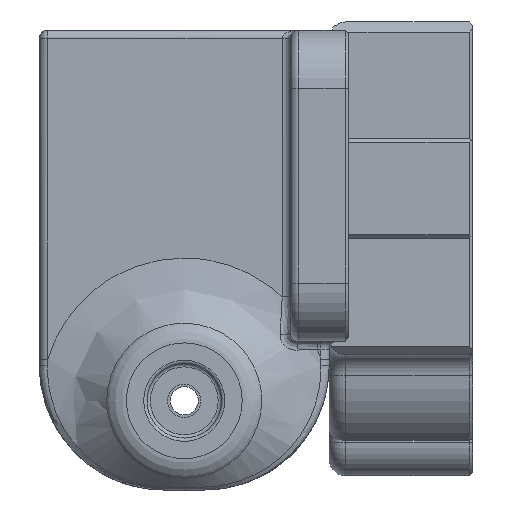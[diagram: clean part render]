
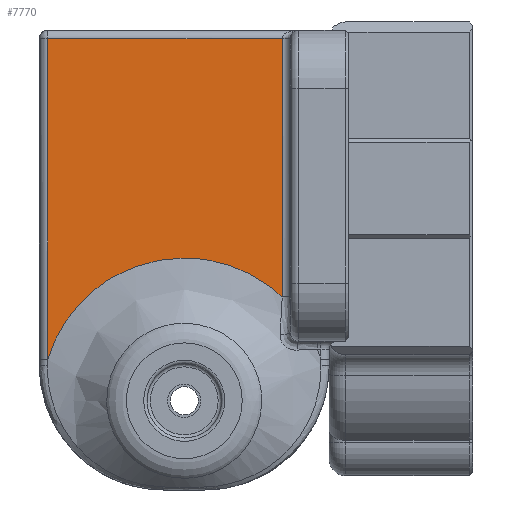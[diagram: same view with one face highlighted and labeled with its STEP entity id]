
A CAD part, front view. The second image highlights one B-rep face of the part: STEP entity #7770.
In plain terms, the highlighted planar face has unit normal (0, -1, 0).
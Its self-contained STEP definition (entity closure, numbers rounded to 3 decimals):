
#4 = EDGE_CURVE ( 'NONE', #7866, #7392, #4444, .T. ) ;
#125 = DIRECTION ( 'NONE',  ( 0., 0., 1. ) ) ;
#129 = LINE ( 'NONE', #6286, #3605 ) ;
#166 = B_SPLINE_CURVE_WITH_KNOTS ( 'NONE', 3,
 ( #6291, #770, #1392, #2013, #3269, #1982 ),
 .UNSPECIFIED., .F., .F.,
 ( 4, 1, 1, 4 ),
 ( -1.112, -0.768, -0.383, 0.001 ),
 .UNSPECIFIED. ) ;
#268 = DIRECTION ( 'NONE',  ( 0., 0., -1. ) ) ;
#488 = VERTEX_POINT ( 'NONE', #605 ) ;
#605 = CARTESIAN_POINT ( 'NONE',  ( -230.016, -0.918, 19.1 ) ) ;
#711 = DIRECTION ( 'NONE',  ( 0., 1., 0. ) ) ;
#770 = CARTESIAN_POINT ( 'NONE',  ( -204.019, -0.918, -10.226 ) ) ;
#774 = CARTESIAN_POINT ( 'NONE',  ( -222.019, -0.918, -9.62 ) ) ;
#786 = FACE_OUTER_BOUND ( 'NONE', #4139, .T. ) ;
#806 = CARTESIAN_POINT ( 'NONE',  ( -216.108, -0.918, -7.422 ) ) ;
#921 = CARTESIAN_POINT ( 'NONE',  ( -201.682, -0.918, 19.1 ) ) ;
#1008 = ORIENTED_EDGE ( 'NONE', *, *, #7106, .F. ) ;
#1229 = EDGE_CURVE ( 'NONE', #7392, #1344, #7686, .T. ) ;
#1278 = DIRECTION ( 'NONE',  ( -1., 0., 0. ) ) ;
#1291 = VERTEX_POINT ( 'NONE', #7319 ) ;
#1344 = VERTEX_POINT ( 'NONE', #6747 ) ;
#1392 = CARTESIAN_POINT ( 'NONE',  ( -206.115, -0.918, -8.942 ) ) ;
#1719 = CARTESIAN_POINT ( 'NONE',  ( -225.172, -0.918, -11.883 ) ) ;
#1823 = CARTESIAN_POINT ( 'NONE',  ( -230.014, -0.918, -19.646 ) ) ;
#1982 = CARTESIAN_POINT ( 'NONE',  ( -213.533, -0.918, -7.42 ) ) ;
#2013 = CARTESIAN_POINT ( 'NONE',  ( -209.663, -0.918, -7.708 ) ) ;
#2102 = CARTESIAN_POINT ( 'NONE',  ( -201.682, -0.918, 8.994 ) ) ;
#2452 = CARTESIAN_POINT ( 'NONE',  ( -223.933, -0.918, -10.924 ) ) ;
#2683 = CARTESIAN_POINT ( 'NONE',  ( -223.011, -0.918, -10.226 ) ) ;
#3020 = CARTESIAN_POINT ( 'NONE',  ( -224.042, -0.918, -11.007 ) ) ;
#3093 = ORIENTED_EDGE ( 'NONE', *, *, #7753, .F. ) ;
#3113 = CARTESIAN_POINT ( 'NONE',  ( -201.682, -0.918, -12.122 ) ) ;
#3269 = CARTESIAN_POINT ( 'NONE',  ( -212.247, -0.918, -7.419 ) ) ;
#3275 = LINE ( 'NONE', #2102, #5748 ) ;
#3421 = CARTESIAN_POINT ( 'NONE',  ( -213.533, -0.918, -7.42 ) ) ;
#3543 = CARTESIAN_POINT ( 'NONE',  ( -229.378, -0.918, -17.565 ) ) ;
#3586 = ORIENTED_EDGE ( 'NONE', *, *, #1229, .F. ) ;
#3605 = VECTOR ( 'NONE', #125, 1000. ) ;
#3627 = DIRECTION ( 'NONE',  ( 1., 0., 0. ) ) ;
#3890 = VERTEX_POINT ( 'NONE', #921 ) ;
#4108 = ORIENTED_EDGE ( 'NONE', *, *, #4, .F. ) ;
#4139 = EDGE_LOOP ( 'NONE', ( #4425, #5454, #3093, #3586, #4108, #1008, #6255 ) ) ;
#4283 = EDGE_CURVE ( 'NONE', #1291, #7085, #7699, .T. ) ;
#4379 = CARTESIAN_POINT ( 'NONE',  ( -203.098, -0.918, -10.924 ) ) ;
#4425 = ORIENTED_EDGE ( 'NONE', *, *, #6839, .F. ) ;
#4444 = B_SPLINE_CURVE_WITH_KNOTS ( 'NONE', 3,
 ( #7553, #806, #4451, #774, #2683, #5092 ),
 .UNSPECIFIED., .F., .F.,
 ( 4, 2, 4 ),
 ( 0.002, 0.771, 1.115 ),
 .UNSPECIFIED. ) ;
#4451 = CARTESIAN_POINT ( 'NONE',  ( -218.658, -0.918, -8.005 ) ) ;
#4852 = CARTESIAN_POINT ( 'NONE',  ( -228.349, -0.918, -15.606 ) ) ;
#4931 = CARTESIAN_POINT ( 'NONE',  ( -202.605, -0.918, -11.298 ) ) ;
#5059 = CARTESIAN_POINT ( 'NONE',  ( -203.098, -0.918, -10.924 ) ) ;
#5092 = CARTESIAN_POINT ( 'NONE',  ( -223.933, -0.918, -10.924 ) ) ;
#5295 = LINE ( 'NONE', #5438, #6354 ) ;
#5408 = CARTESIAN_POINT ( 'NONE',  ( -226.188, -0.918, -12.897 ) ) ;
#5438 = CARTESIAN_POINT ( 'NONE',  ( -213.516, -0.918, 19.1 ) ) ;
#5454 = ORIENTED_EDGE ( 'NONE', *, *, #6312, .F. ) ;
#5591 = PLANE ( 'NONE',  #5992 ) ;
#5748 = VECTOR ( 'NONE', #268, 1000. ) ;
#5848 = CARTESIAN_POINT ( 'NONE',  ( -223.933, -0.918, -10.924 ) ) ;
#5992 = AXIS2_PLACEMENT_3D ( 'NONE', #7442, #711, #1278 ) ;
#6255 = ORIENTED_EDGE ( 'NONE', *, *, #4283, .F. ) ;
#6286 = CARTESIAN_POINT ( 'NONE',  ( -230.016, -0.918, -5.442 ) ) ;
#6291 = CARTESIAN_POINT ( 'NONE',  ( -203.098, -0.918, -10.924 ) ) ;
#6312 = EDGE_CURVE ( 'NONE', #488, #3890, #5295, .T. ) ;
#6354 = VECTOR ( 'NONE', #3627, 1000. ) ;
#6747 = CARTESIAN_POINT ( 'NONE',  ( -230.014, -0.918, -19.646 ) ) ;
#6789 = CARTESIAN_POINT ( 'NONE',  ( -202.132, -0.918, -11.698 ) ) ;
#6839 = EDGE_CURVE ( 'NONE', #3890, #1291, #3275, .T. ) ;
#7085 = VERTEX_POINT ( 'NONE', #5059 ) ;
#7106 = EDGE_CURVE ( 'NONE', #7085, #7866, #166, .T. ) ;
#7319 = CARTESIAN_POINT ( 'NONE',  ( -201.682, -0.918, -12.122 ) ) ;
#7392 = VERTEX_POINT ( 'NONE', #5848 ) ;
#7442 = CARTESIAN_POINT ( 'NONE',  ( -213.516, -0.918, -5.442 ) ) ;
#7553 = CARTESIAN_POINT ( 'NONE',  ( -213.533, -0.918, -7.42 ) ) ;
#7686 = B_SPLINE_CURVE_WITH_KNOTS ( 'NONE', 3,
 ( #2452, #3020, #1719, #5408, #4852, #3543, #1823 ),
 .UNSPECIFIED., .F., .F.,
 ( 4, 1, 2, 4 ),
 ( 1.115, 1.156, 1.54, 2.189 ),
 .UNSPECIFIED. ) ;
#7699 = B_SPLINE_CURVE_WITH_KNOTS ( 'NONE', 3,
 ( #3113, #6789, #4931, #4379 ),
 .UNSPECIFIED., .F., .F.,
 ( 4, 4 ),
 ( -1.296, -1.112 ),
 .UNSPECIFIED. ) ;
#7753 = EDGE_CURVE ( 'NONE', #1344, #488, #129, .T. ) ;
#7770 = ADVANCED_FACE ( 'NONE', ( #786 ), #5591, .F. ) ;
#7866 = VERTEX_POINT ( 'NONE', #3421 ) ;
